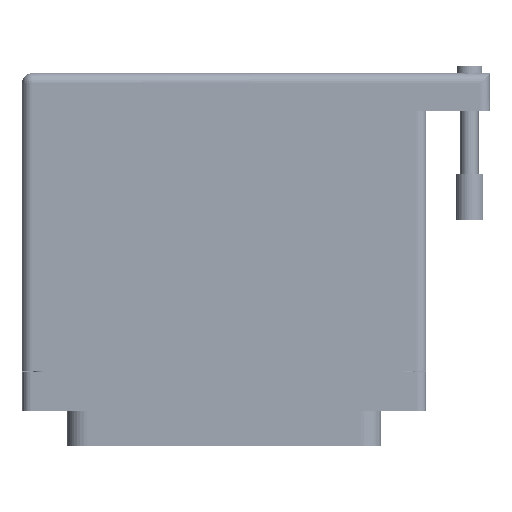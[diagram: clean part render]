
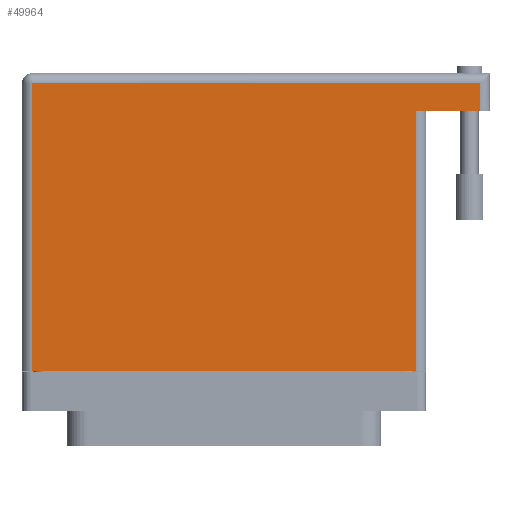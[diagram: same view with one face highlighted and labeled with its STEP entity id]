
A CAD part, front view. The second image highlights one B-rep face of the part: STEP entity #49964.
In plain terms, the highlighted face is planar.
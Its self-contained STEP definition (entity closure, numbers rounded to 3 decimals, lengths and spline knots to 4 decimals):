
#2500 = EDGE_CURVE ( 'NONE', #2851, #88772, #27448, .T. ) ;
#2851 = VERTEX_POINT ( 'NONE', #17397 ) ;
#4693 = DIRECTION ( 'NONE',  ( 0., 1., 0. ) ) ;
#6843 = LINE ( 'NONE', #74536, #80694 ) ;
#8856 = CARTESIAN_POINT ( 'NONE',  ( -1.3775, 1.93, 0.765 ) ) ;
#10724 = CARTESIAN_POINT ( 'NONE',  ( -1.3075, 1.86, 0.765 ) ) ;
#11383 = VERTEX_POINT ( 'NONE', #26125 ) ;
#16042 = DIRECTION ( 'NONE',  ( 1., 0., 0. ) ) ;
#16896 = VECTOR ( 'NONE', #41975, 39.3701 ) ;
#17397 = CARTESIAN_POINT ( 'NONE',  ( 1.7425, 1.86, 0.765 ) ) ;
#17931 = LINE ( 'NONE', #61604, #91766 ) ;
#23481 = ORIENTED_EDGE ( 'NONE', *, *, #57985, .T. ) ;
#25795 = LINE ( 'NONE', #43573, #63936 ) ;
#26125 = CARTESIAN_POINT ( 'NONE',  ( -1.3075, -0.1, 0.765 ) ) ;
#27448 = LINE ( 'NONE', #90325, #57683 ) ;
#29047 = CARTESIAN_POINT ( 'NONE',  ( 1.3075, -0.1, 0.765 ) ) ;
#32540 = LINE ( 'NONE', #40446, #16896 ) ;
#34019 = DIRECTION ( 'NONE',  ( 0., 1., 0. ) ) ;
#35087 = EDGE_CURVE ( 'NONE', #52861, #90957, #17931, .T. ) ;
#40054 = VECTOR ( 'NONE', #4693, 39.3701 ) ;
#40446 = CARTESIAN_POINT ( 'NONE',  ( 1.8125, 1.674, 0.765 ) ) ;
#41396 = EDGE_CURVE ( 'NONE', #82337, #90957, #32540, .T. ) ;
#41975 = DIRECTION ( 'NONE',  ( -1., 0., 0. ) ) ;
#43181 = EDGE_CURVE ( 'NONE', #82337, #2851, #88141, .T. ) ;
#43573 = CARTESIAN_POINT ( 'NONE',  ( -1.3775, -0.1, 0.765 ) ) ;
#48096 = FACE_OUTER_BOUND ( 'NONE', #89384, .T. ) ;
#48967 = ORIENTED_EDGE ( 'NONE', *, *, #35087, .T. ) ;
#49964 = ADVANCED_FACE ( 'NONE', ( #48096 ), #52042, .F. ) ;
#52042 = PLANE ( 'NONE',  #79154 ) ;
#52861 = VERTEX_POINT ( 'NONE', #29047 ) ;
#55036 = DIRECTION ( 'NONE',  ( -1., 0., 0. ) ) ;
#57683 = VECTOR ( 'NONE', #55036, 39.3701 ) ;
#57985 = EDGE_CURVE ( 'NONE', #88772, #11383, #6843, .T. ) ;
#58915 = DIRECTION ( 'NONE',  ( 0., 0., -1. ) ) ;
#61604 = CARTESIAN_POINT ( 'NONE',  ( 1.3075, 1.674, 0.765 ) ) ;
#61937 = CARTESIAN_POINT ( 'NONE',  ( 1.7425, 1.93, 0.765 ) ) ;
#63936 = VECTOR ( 'NONE', #16042, 39.3701 ) ;
#66233 = CARTESIAN_POINT ( 'NONE',  ( 1.3075, 1.674, 0.765 ) ) ;
#66398 = DIRECTION ( 'NONE',  ( -1., 0., 0. ) ) ;
#66623 = ORIENTED_EDGE ( 'NONE', *, *, #69069, .T. ) ;
#68846 = ORIENTED_EDGE ( 'NONE', *, *, #2500, .T. ) ;
#69069 = EDGE_CURVE ( 'NONE', #11383, #52861, #25795, .T. ) ;
#70700 = ORIENTED_EDGE ( 'NONE', *, *, #41396, .F. ) ;
#74536 = CARTESIAN_POINT ( 'NONE',  ( -1.3075, -0.1, 0.765 ) ) ;
#75728 = DIRECTION ( 'NONE',  ( 0., -1., 0. ) ) ;
#79154 = AXIS2_PLACEMENT_3D ( 'NONE', #8856, #58915, #66398 ) ;
#79332 = CARTESIAN_POINT ( 'NONE',  ( 1.7425, 1.674, 0.765 ) ) ;
#80694 = VECTOR ( 'NONE', #75728, 39.3701 ) ;
#82337 = VERTEX_POINT ( 'NONE', #79332 ) ;
#86065 = ORIENTED_EDGE ( 'NONE', *, *, #43181, .T. ) ;
#88141 = LINE ( 'NONE', #61937, #40054 ) ;
#88772 = VERTEX_POINT ( 'NONE', #10724 ) ;
#89384 = EDGE_LOOP ( 'NONE', ( #66623, #48967, #70700, #86065, #68846, #23481 ) ) ;
#90325 = CARTESIAN_POINT ( 'NONE',  ( -1.3775, 1.86, 0.765 ) ) ;
#90957 = VERTEX_POINT ( 'NONE', #66233 ) ;
#91766 = VECTOR ( 'NONE', #34019, 39.3701 ) ;
